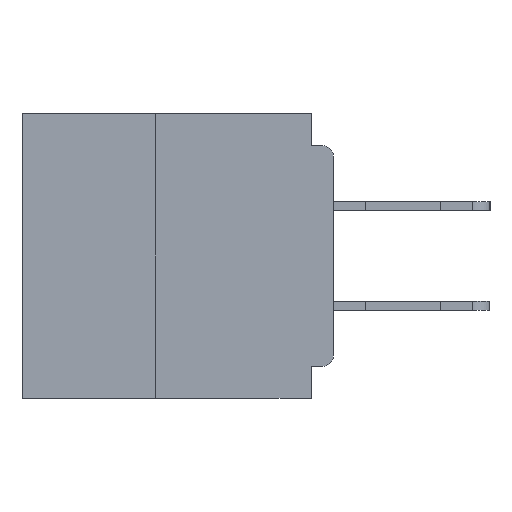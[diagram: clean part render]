
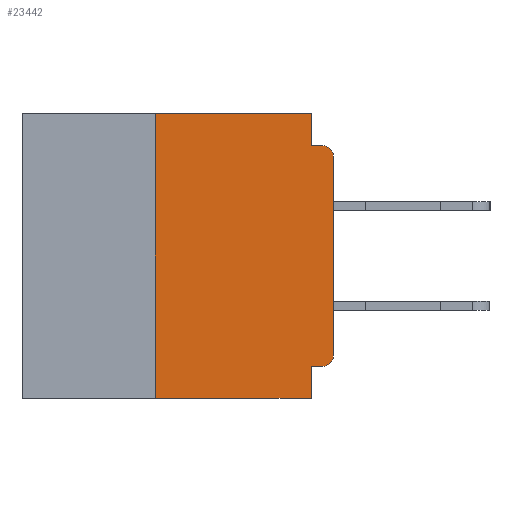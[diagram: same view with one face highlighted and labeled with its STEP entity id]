
A CAD part, left-side view. The second image highlights one B-rep face of the part: STEP entity #23442.
In plain terms, the highlighted planar face has unit normal (-1, 0, 0).
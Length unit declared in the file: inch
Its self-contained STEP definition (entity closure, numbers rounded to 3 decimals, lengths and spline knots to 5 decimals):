
#115 = CARTESIAN_POINT ( 'NONE',  ( 0., 0.031, 0. ) ) ;
#556 = VERTEX_POINT ( 'NONE', #115 ) ;
#835 = EDGE_CURVE ( 'NONE', #34513, #25524, #13035, .T. ) ;
#924 = AXIS2_PLACEMENT_3D ( 'NONE', #27073, #8795, #30100 ) ;
#1029 = VECTOR ( 'NONE', #31085, 39.37008 ) ;
#2837 = LINE ( 'NONE', #11941, #34329 ) ;
#3344 = ORIENTED_EDGE ( 'NONE', *, *, #16898, .T. ) ;
#4515 = CARTESIAN_POINT ( 'NONE',  ( 0., 0.25, -0.4 ) ) ;
#4794 = VECTOR ( 'NONE', #36325, 39.37008 ) ;
#4853 = ORIENTED_EDGE ( 'NONE', *, *, #835, .F. ) ;
#4996 = CARTESIAN_POINT ( 'NONE',  ( 0., 0.031, -0.4 ) ) ;
#5796 = CARTESIAN_POINT ( 'NONE',  ( 0., 0.031, -0.4 ) ) ;
#5817 = ORIENTED_EDGE ( 'NONE', *, *, #20228, .F. ) ;
#5824 = DIRECTION ( 'NONE',  ( 0., -1., 0. ) ) ;
#5849 = VERTEX_POINT ( 'NONE', #31096 ) ;
#6053 = FACE_OUTER_BOUND ( 'NONE', #20990, .T. ) ;
#6111 = VERTEX_POINT ( 'NONE', #4515 ) ;
#6694 = CARTESIAN_POINT ( 'NONE',  ( 0., 0., -0.045 ) ) ;
#7079 = EDGE_CURVE ( 'NONE', #26435, #12581, #28817, .T. ) ;
#8568 = CARTESIAN_POINT ( 'NONE',  ( 0., 0.437, 0. ) ) ;
#8795 = DIRECTION ( 'NONE',  ( -1., 0., 0. ) ) ;
#9742 = AXIS2_PLACEMENT_3D ( 'NONE', #8568, #38780, #20937 ) ;
#10211 = ORIENTED_EDGE ( 'NONE', *, *, #28402, .F. ) ;
#10252 = VECTOR ( 'NONE', #36236, 39.37008 ) ;
#11151 = CARTESIAN_POINT ( 'NONE',  ( 0., 0.25, -0.4 ) ) ;
#11941 = CARTESIAN_POINT ( 'NONE',  ( 0., 0.437, 0. ) ) ;
#12069 = VERTEX_POINT ( 'NONE', #37432 ) ;
#12115 = CARTESIAN_POINT ( 'NONE',  ( 0., 0.031, 0. ) ) ;
#12221 = VECTOR ( 'NONE', #27852, 39.37008 ) ;
#12581 = VERTEX_POINT ( 'NONE', #37404 ) ;
#13035 = LINE ( 'NONE', #5796, #4794 ) ;
#13530 = DIRECTION ( 'NONE',  ( -1., 0., 0. ) ) ;
#16708 = LINE ( 'NONE', #31760, #25734 ) ;
#16868 = CIRCLE ( 'NONE', #28810, 0.015 ) ;
#16875 = DIRECTION ( 'NONE',  ( 0., -1., 0. ) ) ;
#16898 = EDGE_CURVE ( 'NONE', #12581, #22737, #28404, .T. ) ;
#19309 = ORIENTED_EDGE ( 'NONE', *, *, #34384, .T. ) ;
#19353 = LINE ( 'NONE', #12115, #10252 ) ;
#19681 = VECTOR ( 'NONE', #20379, 39.37008 ) ;
#20174 = CARTESIAN_POINT ( 'NONE',  ( 0., 0.031, -0.045 ) ) ;
#20228 = EDGE_CURVE ( 'NONE', #26435, #34513, #16708, .T. ) ;
#20294 = VERTEX_POINT ( 'NONE', #20174 ) ;
#20379 = DIRECTION ( 'NONE',  ( 0., 0., 1. ) ) ;
#20937 = DIRECTION ( 'NONE',  ( 0., 0., -1. ) ) ;
#20990 = EDGE_LOOP ( 'NONE', ( #3344, #36643, #21695, #23601, #39374, #10211, #19309, #4853, #5817, #22211 ) ) ;
#21608 = CARTESIAN_POINT ( 'NONE',  ( 0., 0.015, -0.355 ) ) ;
#21695 = ORIENTED_EDGE ( 'NONE', *, *, #31073, .F. ) ;
#22139 = LINE ( 'NONE', #37856, #23077 ) ;
#22211 = ORIENTED_EDGE ( 'NONE', *, *, #7079, .T. ) ;
#22737 = VERTEX_POINT ( 'NONE', #38458 ) ;
#23077 = VECTOR ( 'NONE', #16875, 39.37008 ) ;
#23442 = ADVANCED_FACE ( 'NONE', ( #6053 ), #32887, .F. ) ;
#23601 = ORIENTED_EDGE ( 'NONE', *, *, #26370, .F. ) ;
#24657 = LINE ( 'NONE', #6694, #1029 ) ;
#24838 = CARTESIAN_POINT ( 'NONE',  ( 0., 0., 0. ) ) ;
#25524 = VERTEX_POINT ( 'NONE', #4996 ) ;
#25734 = VECTOR ( 'NONE', #34736, 39.37008 ) ;
#26370 = EDGE_CURVE ( 'NONE', #556, #20294, #19353, .T. ) ;
#26435 = VERTEX_POINT ( 'NONE', #21608 ) ;
#27073 = CARTESIAN_POINT ( 'NONE',  ( 0., 0.015, -0.34 ) ) ;
#27701 = LINE ( 'NONE', #11151, #19681 ) ;
#27852 = DIRECTION ( 'NONE',  ( 0., 0., 1. ) ) ;
#28402 = EDGE_CURVE ( 'NONE', #6111, #5849, #27701, .T. ) ;
#28404 = LINE ( 'NONE', #24838, #12221 ) ;
#28810 = AXIS2_PLACEMENT_3D ( 'NONE', #31664, #13530, #34644 ) ;
#28817 = CIRCLE ( 'NONE', #924, 0.015 ) ;
#30100 = DIRECTION ( 'NONE',  ( 0., 0., -1. ) ) ;
#31073 = EDGE_CURVE ( 'NONE', #20294, #12069, #24657, .T. ) ;
#31085 = DIRECTION ( 'NONE',  ( 0., -1., 0. ) ) ;
#31096 = CARTESIAN_POINT ( 'NONE',  ( 0., 0.25, 0. ) ) ;
#31664 = CARTESIAN_POINT ( 'NONE',  ( 0., 0.015, -0.06 ) ) ;
#31760 = CARTESIAN_POINT ( 'NONE',  ( 0., 0., -0.355 ) ) ;
#32887 = PLANE ( 'NONE',  #9742 ) ;
#34047 = EDGE_CURVE ( 'NONE', #5849, #556, #2837, .T. ) ;
#34314 = EDGE_CURVE ( 'NONE', #22737, #12069, #16868, .T. ) ;
#34329 = VECTOR ( 'NONE', #5824, 39.37008 ) ;
#34384 = EDGE_CURVE ( 'NONE', #6111, #25524, #22139, .T. ) ;
#34513 = VERTEX_POINT ( 'NONE', #35538 ) ;
#34644 = DIRECTION ( 'NONE',  ( 0., 0., -1. ) ) ;
#34736 = DIRECTION ( 'NONE',  ( 0., 1., 0. ) ) ;
#35538 = CARTESIAN_POINT ( 'NONE',  ( 0., 0.031, -0.355 ) ) ;
#36236 = DIRECTION ( 'NONE',  ( 0., 0., -1. ) ) ;
#36325 = DIRECTION ( 'NONE',  ( 0., 0., -1. ) ) ;
#36643 = ORIENTED_EDGE ( 'NONE', *, *, #34314, .T. ) ;
#37404 = CARTESIAN_POINT ( 'NONE',  ( 0., 0., -0.34 ) ) ;
#37432 = CARTESIAN_POINT ( 'NONE',  ( 0., 0.015, -0.045 ) ) ;
#37856 = CARTESIAN_POINT ( 'NONE',  ( 0., 0.437, -0.4 ) ) ;
#38458 = CARTESIAN_POINT ( 'NONE',  ( 0., 0., -0.06 ) ) ;
#38780 = DIRECTION ( 'NONE',  ( 1., 0., 0. ) ) ;
#39374 = ORIENTED_EDGE ( 'NONE', *, *, #34047, .F. ) ;
